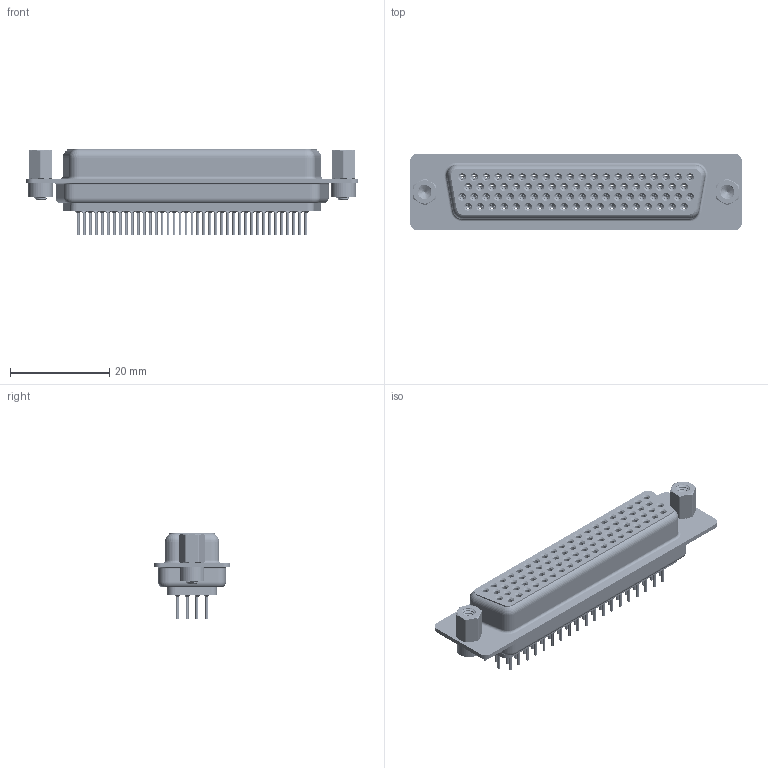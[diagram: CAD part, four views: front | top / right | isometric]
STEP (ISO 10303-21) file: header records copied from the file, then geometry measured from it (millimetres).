
FILE_DESCRIPTION (( 'STEP AP203' ), '1' );
FILE_NAME ('638-078-630-243.STEP', '2020-07-20T04:35:16', ( '' ), ( '' ), 'SwSTEP 2.0', 'SolidWorks 2020', '' );
FILE_SCHEMA (( 'CONFIG_CONTROL_DESIGN' ));
Length unit declared in the file: millimetre
Products named in the file (10): 638 Shell Rear_78 Contacts; 638-078-630-243; 638 4-40 Threaded Rivet; 638 Contact Row 1_30; 638 Contact Row 78_30; 638 4-40 Hex Standoff; 638 Contact Row 3_30; 638 Shell Front_78 Contacts; 638 Contact Row 2_30; 638 Housing_78 Contacts
Assembly tree (85 placements, depth 2):
  638-078-630-243
    638 Housing_78 Contacts
    638 Shell Front_78 Contacts
    638 Shell Rear_78 Contacts
    638 Contact Row 1_30  x19
    638 Contact Row 2_30  x20
    638 Contact Row 3_30  x19
    638 Contact Row 78_30  x20
    638 4-40 Threaded Rivet  x2
    638 4-40 Hex Standoff  x2
Bounding box: 67 x 15.4 x 17.3 mm (x, y, z)
Volume: 6088.3 mm3; surface area: 21006.9 mm2
Topology: 85 solids, 85 shells, 10311 faces, 26265 edges, 16291 vertices
Faces by surface type: cylinder 2783, plane 2507, torus 2125, bspline 1578, cone 1318
Entity records: 62527 total; most frequent: CARTESIAN_POINT 17890, DIRECTION 9249, ORIENTED_EDGE 8252, EDGE_CURVE 4126, AXIS2_PLACEMENT_3D 3915, VERTEX_POINT 2616, EDGE_LOOP 2188, CIRCLE 2143
